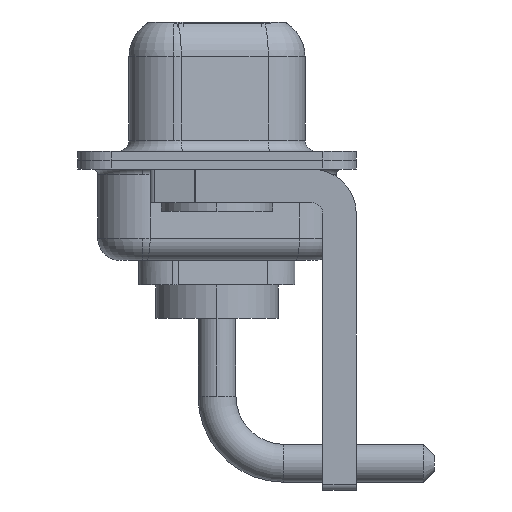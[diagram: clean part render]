
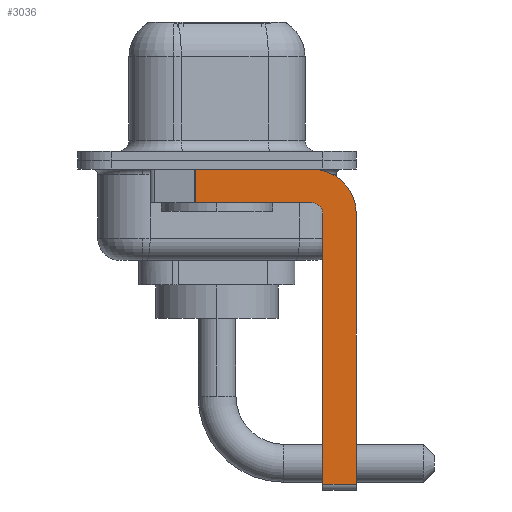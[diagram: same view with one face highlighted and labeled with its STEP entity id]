
A CAD part, left-side view. The second image highlights one B-rep face of the part: STEP entity #3036.
In plain terms, the highlighted planar face has unit normal (-1, 0, 0).
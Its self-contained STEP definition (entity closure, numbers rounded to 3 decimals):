
#154 = VECTOR ( 'NONE', #4581, 1000. ) ;
#194 = CARTESIAN_POINT ( 'NONE',  ( -2.9, -4.75, -14.8 ) ) ;
#405 = CARTESIAN_POINT ( 'NONE',  ( -2.9, -4.25, -1.9 ) ) ;
#453 = EDGE_CURVE ( 'NONE', #1296, #7253, #1943, .T. ) ;
#560 = VERTEX_POINT ( 'NONE', #669 ) ;
#617 = CARTESIAN_POINT ( 'NONE',  ( -2.9, -4.75, -14.55 ) ) ;
#669 = CARTESIAN_POINT ( 'NONE',  ( -2.9, 0.978, -1.9 ) ) ;
#1244 = CARTESIAN_POINT ( 'NONE',  ( -2.9, -4.25, -2.4 ) ) ;
#1296 = VERTEX_POINT ( 'NONE', #9514 ) ;
#1532 = VERTEX_POINT ( 'NONE', #5219 ) ;
#1592 = CARTESIAN_POINT ( 'NONE',  ( -2.9, 0.978, -1.9 ) ) ;
#1943 = CIRCLE ( 'NONE', #2374, 2. ) ;
#2239 = VERTEX_POINT ( 'NONE', #617 ) ;
#2374 = AXIS2_PLACEMENT_3D ( 'NONE', #3427, #5580, #12744 ) ;
#2431 = ORIENTED_EDGE ( 'NONE', *, *, #3671, .T. ) ;
#2666 = CARTESIAN_POINT ( 'NONE',  ( -2.9, -6.25, -14.55 ) ) ;
#2913 = VECTOR ( 'NONE', #7711, 1000. ) ;
#3036 = ADVANCED_FACE ( 'NONE', ( #12724 ), #12789, .F. ) ;
#3275 = DIRECTION ( 'NONE',  ( 0., 0., -1. ) ) ;
#3427 = CARTESIAN_POINT ( 'NONE',  ( -2.9, -4.25, -2.4 ) ) ;
#3671 = EDGE_CURVE ( 'NONE', #9585, #560, #10940, .T. ) ;
#4002 = ORIENTED_EDGE ( 'NONE', *, *, #5897, .F. ) ;
#4075 = ORIENTED_EDGE ( 'NONE', *, *, #12858, .F. ) ;
#4153 = ORIENTED_EDGE ( 'NONE', *, *, #453, .F. ) ;
#4241 = VECTOR ( 'NONE', #8149, 1000. ) ;
#4312 = CARTESIAN_POINT ( 'NONE',  ( -2.9, 3., -0.4 ) ) ;
#4342 = EDGE_CURVE ( 'NONE', #7253, #5145, #7247, .T. ) ;
#4384 = DIRECTION ( 'NONE',  ( -1., 0., 0. ) ) ;
#4581 = DIRECTION ( 'NONE',  ( 0., 1., 0. ) ) ;
#4958 = CARTESIAN_POINT ( 'NONE',  ( -2.9, -4.25, -14.55 ) ) ;
#5145 = VERTEX_POINT ( 'NONE', #2666 ) ;
#5219 = CARTESIAN_POINT ( 'NONE',  ( -2.9, -4.25, -1.9 ) ) ;
#5580 = DIRECTION ( 'NONE',  ( 1., 0., 0. ) ) ;
#5591 = LINE ( 'NONE', #405, #154 ) ;
#5759 = VECTOR ( 'NONE', #7352, 1000. ) ;
#5897 = EDGE_CURVE ( 'NONE', #1532, #560, #5591, .T. ) ;
#6353 = VECTOR ( 'NONE', #11870, 1000. ) ;
#7247 = LINE ( 'NONE', #9444, #4241 ) ;
#7253 = VERTEX_POINT ( 'NONE', #12019 ) ;
#7332 = CARTESIAN_POINT ( 'NONE',  ( -2.9, -4.75, -2.4 ) ) ;
#7333 = CARTESIAN_POINT ( 'NONE',  ( -2.9, -4.25, -2.4 ) ) ;
#7352 = DIRECTION ( 'NONE',  ( 0., 0., 1. ) ) ;
#7711 = DIRECTION ( 'NONE',  ( 0., 0., -1. ) ) ;
#8149 = DIRECTION ( 'NONE',  ( 0., 0., -1. ) ) ;
#8519 = LINE ( 'NONE', #194, #5759 ) ;
#8922 = EDGE_CURVE ( 'NONE', #9585, #1296, #11602, .T. ) ;
#8925 = LINE ( 'NONE', #4958, #10989 ) ;
#9072 = EDGE_LOOP ( 'NONE', ( #10128, #2431, #4002, #4075, #10220, #9494, #11558, #4153 ) ) ;
#9444 = CARTESIAN_POINT ( 'NONE',  ( -2.9, -6.25, -2.4 ) ) ;
#9494 = ORIENTED_EDGE ( 'NONE', *, *, #12318, .T. ) ;
#9514 = CARTESIAN_POINT ( 'NONE',  ( -2.9, -4.25, -0.4 ) ) ;
#9524 = VERTEX_POINT ( 'NONE', #7332 ) ;
#9585 = VERTEX_POINT ( 'NONE', #11040 ) ;
#10128 = ORIENTED_EDGE ( 'NONE', *, *, #8922, .F. ) ;
#10220 = ORIENTED_EDGE ( 'NONE', *, *, #11610, .F. ) ;
#10506 = DIRECTION ( 'NONE',  ( 1., 0., 0. ) ) ;
#10721 = DIRECTION ( 'NONE',  ( 0., 0., 1. ) ) ;
#10940 = LINE ( 'NONE', #1592, #2913 ) ;
#10989 = VECTOR ( 'NONE', #11180, 1000. ) ;
#11040 = CARTESIAN_POINT ( 'NONE',  ( -2.9, 0.978, -0.4 ) ) ;
#11180 = DIRECTION ( 'NONE',  ( 0., -1., 0. ) ) ;
#11558 = ORIENTED_EDGE ( 'NONE', *, *, #4342, .F. ) ;
#11602 = LINE ( 'NONE', #4312, #6353 ) ;
#11610 = EDGE_CURVE ( 'NONE', #2239, #9524, #8519, .T. ) ;
#11870 = DIRECTION ( 'NONE',  ( 0., -1., 0. ) ) ;
#12019 = CARTESIAN_POINT ( 'NONE',  ( -2.9, -6.25, -2.4 ) ) ;
#12083 = CIRCLE ( 'NONE', #12502, 0.5 ) ;
#12318 = EDGE_CURVE ( 'NONE', #2239, #5145, #8925, .T. ) ;
#12442 = AXIS2_PLACEMENT_3D ( 'NONE', #7333, #10506, #3275 ) ;
#12502 = AXIS2_PLACEMENT_3D ( 'NONE', #1244, #4384, #10721 ) ;
#12724 = FACE_OUTER_BOUND ( 'NONE', #9072, .T. ) ;
#12744 = DIRECTION ( 'NONE',  ( 0., 0., -1. ) ) ;
#12789 = PLANE ( 'NONE',  #12442 ) ;
#12858 = EDGE_CURVE ( 'NONE', #9524, #1532, #12083, .T. ) ;
